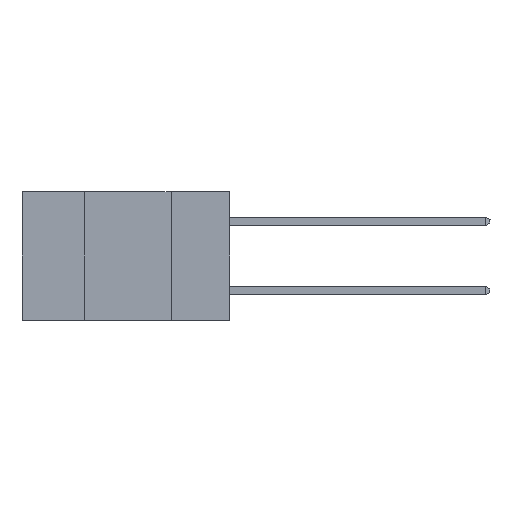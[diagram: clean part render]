
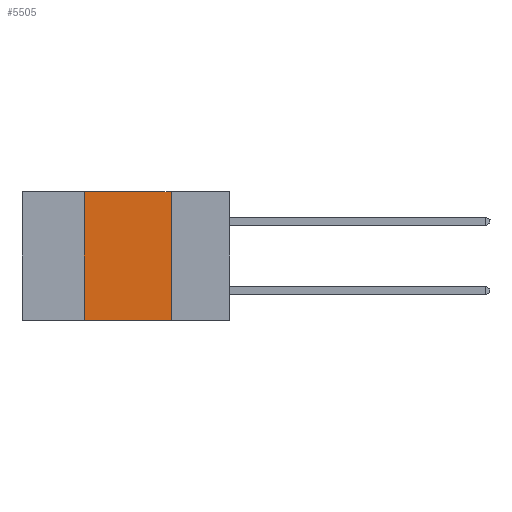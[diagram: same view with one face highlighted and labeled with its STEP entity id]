
A CAD part, left-side view. The second image highlights one B-rep face of the part: STEP entity #5505.
In plain terms, the highlighted planar face has unit normal (-1, 0, 0).
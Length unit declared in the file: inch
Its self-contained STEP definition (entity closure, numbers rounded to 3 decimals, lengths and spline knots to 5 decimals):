
#97 = LINE ( 'NONE', #10669, #5180 ) ;
#292 = FACE_OUTER_BOUND ( 'NONE', #12282, .T. ) ;
#1399 = VERTEX_POINT ( 'NONE', #8860 ) ;
#1694 = EDGE_CURVE ( 'NONE', #10793, #6271, #7628, .T. ) ;
#2349 = DIRECTION ( 'NONE',  ( 0., -1., 0. ) ) ;
#2857 = EDGE_CURVE ( 'NONE', #1399, #6261, #6948, .T. ) ;
#2901 = AXIS2_PLACEMENT_3D ( 'NONE', #10811, #3224, #4222 ) ;
#3224 = DIRECTION ( 'NONE',  ( 1., 0., 0. ) ) ;
#3400 = ORIENTED_EDGE ( 'NONE', *, *, #1694, .T. ) ;
#3602 = CARTESIAN_POINT ( 'NONE',  ( 0., 0.6, -0.37 ) ) ;
#3655 = EDGE_CURVE ( 'NONE', #6261, #6271, #97, .T. ) ;
#3920 = LINE ( 'NONE', #4737, #8984 ) ;
#4090 = PLANE ( 'NONE',  #2901 ) ;
#4222 = DIRECTION ( 'NONE',  ( 0., 0., -1. ) ) ;
#4291 = CARTESIAN_POINT ( 'NONE',  ( 0., 0.6, 0. ) ) ;
#4662 = DIRECTION ( 'NONE',  ( 0., -1., 0. ) ) ;
#4737 = CARTESIAN_POINT ( 'NONE',  ( 0., 0.42, -0.37 ) ) ;
#4765 = CARTESIAN_POINT ( 'NONE',  ( 0., 0.17, 0. ) ) ;
#5180 = VECTOR ( 'NONE', #11483, 39.37008 ) ;
#5505 = ADVANCED_FACE ( 'NONE', ( #292 ), #4090, .F. ) ;
#6261 = VERTEX_POINT ( 'NONE', #4765 ) ;
#6271 = VERTEX_POINT ( 'NONE', #9385 ) ;
#6948 = LINE ( 'NONE', #4291, #7287 ) ;
#7287 = VECTOR ( 'NONE', #2349, 39.37008 ) ;
#7628 = LINE ( 'NONE', #3602, #8320 ) ;
#8320 = VECTOR ( 'NONE', #4662, 39.37008 ) ;
#8847 = ORIENTED_EDGE ( 'NONE', *, *, #2857, .F. ) ;
#8860 = CARTESIAN_POINT ( 'NONE',  ( 0., 0.42, 0. ) ) ;
#8984 = VECTOR ( 'NONE', #10580, 39.37008 ) ;
#9125 = ORIENTED_EDGE ( 'NONE', *, *, #3655, .F. ) ;
#9385 = CARTESIAN_POINT ( 'NONE',  ( 0., 0.17, -0.37 ) ) ;
#10483 = CARTESIAN_POINT ( 'NONE',  ( 0., 0.42, -0.37 ) ) ;
#10580 = DIRECTION ( 'NONE',  ( 0., 0., 1. ) ) ;
#10669 = CARTESIAN_POINT ( 'NONE',  ( 0., 0.17, -0.37 ) ) ;
#10793 = VERTEX_POINT ( 'NONE', #10483 ) ;
#10811 = CARTESIAN_POINT ( 'NONE',  ( 0., 0.6, 0. ) ) ;
#11483 = DIRECTION ( 'NONE',  ( 0., 0., -1. ) ) ;
#11599 = EDGE_CURVE ( 'NONE', #10793, #1399, #3920, .T. ) ;
#11952 = ORIENTED_EDGE ( 'NONE', *, *, #11599, .F. ) ;
#12282 = EDGE_LOOP ( 'NONE', ( #9125, #8847, #11952, #3400 ) ) ;
